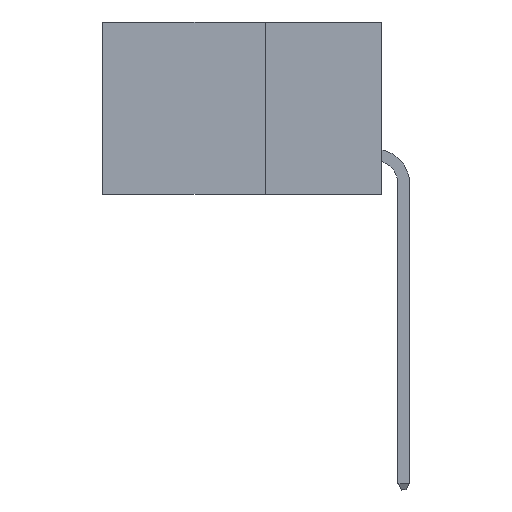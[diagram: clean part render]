
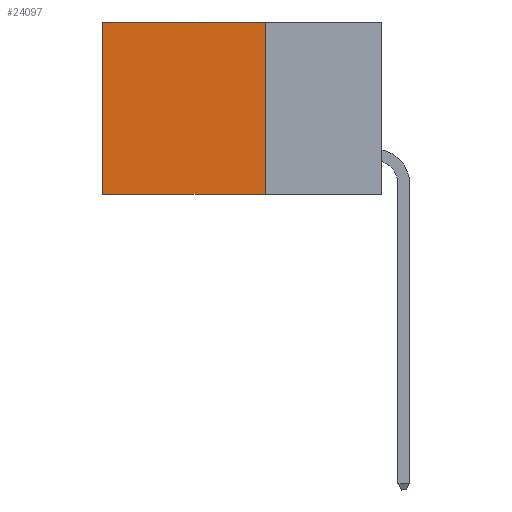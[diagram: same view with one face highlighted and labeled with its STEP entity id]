
A CAD part, left-side view. The second image highlights one B-rep face of the part: STEP entity #24097.
In plain terms, the highlighted planar face has unit normal (-1, 0, 0).
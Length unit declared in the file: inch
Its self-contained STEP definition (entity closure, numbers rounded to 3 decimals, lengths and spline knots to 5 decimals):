
#246 = DIRECTION ( 'NONE',  ( 1., 0., 0. ) ) ;
#976 = VERTEX_POINT ( 'NONE', #27565 ) ;
#1994 = VECTOR ( 'NONE', #17833, 39.37008 ) ;
#2896 = VECTOR ( 'NONE', #9638, 39.37008 ) ;
#3815 = LINE ( 'NONE', #5585, #25258 ) ;
#4233 = ORIENTED_EDGE ( 'NONE', *, *, #12655, .F. ) ;
#4789 = EDGE_CURVE ( 'NONE', #976, #14932, #14617, .T. ) ;
#5585 = CARTESIAN_POINT ( 'NONE',  ( 0.2875, 0.6, 0. ) ) ;
#5861 = VERTEX_POINT ( 'NONE', #8227 ) ;
#8227 = CARTESIAN_POINT ( 'NONE',  ( 0.2875, 0.6, 0. ) ) ;
#9638 = DIRECTION ( 'NONE',  ( 0., 1., 0. ) ) ;
#10993 = CARTESIAN_POINT ( 'NONE',  ( 0.2875, 0.6, -0.37 ) ) ;
#11070 = CARTESIAN_POINT ( 'NONE',  ( 0.2875, 0.25, 0. ) ) ;
#11208 = DIRECTION ( 'NONE',  ( 0., 0., -1. ) ) ;
#12149 = CARTESIAN_POINT ( 'NONE',  ( 0.2875, 0.25, 0. ) ) ;
#12655 = EDGE_CURVE ( 'NONE', #21674, #976, #17865, .T. ) ;
#13314 = CARTESIAN_POINT ( 'NONE',  ( 0.2875, 0.25, 0. ) ) ;
#14617 = LINE ( 'NONE', #16963, #2896 ) ;
#14767 = ORIENTED_EDGE ( 'NONE', *, *, #21299, .T. ) ;
#14932 = VERTEX_POINT ( 'NONE', #10993 ) ;
#16963 = CARTESIAN_POINT ( 'NONE',  ( 0.2875, 0.25, -0.37 ) ) ;
#17833 = DIRECTION ( 'NONE',  ( 0., 0., -1. ) ) ;
#17865 = LINE ( 'NONE', #11070, #1994 ) ;
#17905 = ORIENTED_EDGE ( 'NONE', *, *, #24697, .T. ) ;
#19742 = ORIENTED_EDGE ( 'NONE', *, *, #4789, .F. ) ;
#20303 = EDGE_LOOP ( 'NONE', ( #14767, #19742, #4233, #17905 ) ) ;
#20349 = VECTOR ( 'NONE', #21192, 39.37008 ) ;
#21058 = DIRECTION ( 'NONE',  ( 0., 0., -1. ) ) ;
#21192 = DIRECTION ( 'NONE',  ( 0., 1., 0. ) ) ;
#21299 = EDGE_CURVE ( 'NONE', #5861, #14932, #3815, .T. ) ;
#21674 = VERTEX_POINT ( 'NONE', #12149 ) ;
#22414 = CARTESIAN_POINT ( 'NONE',  ( 0.2875, 0.25, 0. ) ) ;
#22436 = PLANE ( 'NONE',  #27198 ) ;
#23456 = LINE ( 'NONE', #22414, #20349 ) ;
#24097 = ADVANCED_FACE ( 'NONE', ( #26615 ), #22436, .F. ) ;
#24697 = EDGE_CURVE ( 'NONE', #21674, #5861, #23456, .T. ) ;
#25258 = VECTOR ( 'NONE', #21058, 39.37008 ) ;
#26615 = FACE_OUTER_BOUND ( 'NONE', #20303, .T. ) ;
#27198 = AXIS2_PLACEMENT_3D ( 'NONE', #13314, #246, #11208 ) ;
#27565 = CARTESIAN_POINT ( 'NONE',  ( 0.2875, 0.25, -0.37 ) ) ;
